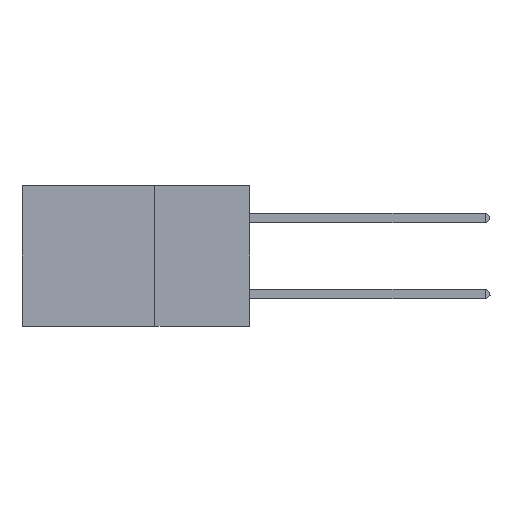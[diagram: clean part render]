
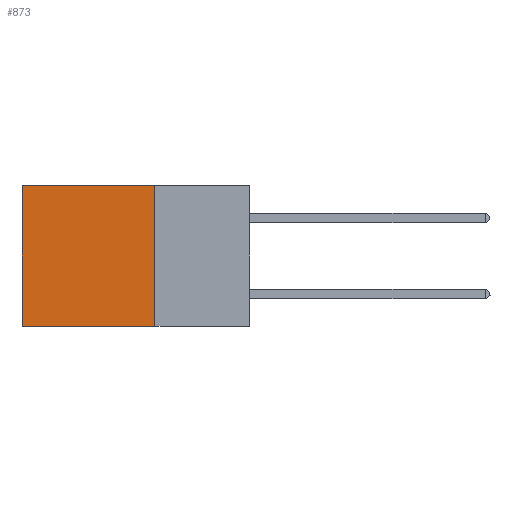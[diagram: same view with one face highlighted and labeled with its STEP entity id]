
A CAD part, left-side view. The second image highlights one B-rep face of the part: STEP entity #873.
In plain terms, the highlighted planar face has unit normal (-1, 0, 0).
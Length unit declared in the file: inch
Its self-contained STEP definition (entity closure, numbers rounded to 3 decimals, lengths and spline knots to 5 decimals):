
#191 = EDGE_LOOP ( 'NONE', ( #27006, #25550, #25940, #15339 ) ) ;
#236 = VECTOR ( 'NONE', #26008, 39.37008 ) ;
#326 = VERTEX_POINT ( 'NONE', #21121 ) ;
#873 = ADVANCED_FACE ( 'NONE', ( #15754 ), #25463, .F. ) ;
#1130 = VECTOR ( 'NONE', #25966, 39.37008 ) ;
#1769 = VECTOR ( 'NONE', #19743, 39.37008 ) ;
#2538 = CARTESIAN_POINT ( 'NONE',  ( 0.2875, 0.25, -0.37 ) ) ;
#9728 = VECTOR ( 'NONE', #25438, 39.37008 ) ;
#10364 = CARTESIAN_POINT ( 'NONE',  ( 0.2875, 0.25, 0. ) ) ;
#10390 = CARTESIAN_POINT ( 'NONE',  ( 0.2875, 0.25, 0. ) ) ;
#10706 = DIRECTION ( 'NONE',  ( 1., 0., 0. ) ) ;
#10878 = LINE ( 'NONE', #10364, #9728 ) ;
#11114 = CARTESIAN_POINT ( 'NONE',  ( 0.2875, 0.25, 0. ) ) ;
#12013 = CARTESIAN_POINT ( 'NONE',  ( 0.2875, 0.6, 0. ) ) ;
#12786 = EDGE_CURVE ( 'NONE', #13239, #17150, #27253, .T. ) ;
#13200 = EDGE_CURVE ( 'NONE', #13239, #31887, #10878, .T. ) ;
#13239 = VERTEX_POINT ( 'NONE', #27892 ) ;
#13364 = CARTESIAN_POINT ( 'NONE',  ( 0.2875, 0.25, -0.37 ) ) ;
#14300 = EDGE_CURVE ( 'NONE', #31887, #326, #20175, .T. ) ;
#15339 = ORIENTED_EDGE ( 'NONE', *, *, #12786, .T. ) ;
#15754 = FACE_OUTER_BOUND ( 'NONE', #191, .T. ) ;
#17150 = VERTEX_POINT ( 'NONE', #21520 ) ;
#19743 = DIRECTION ( 'NONE',  ( 0., 0., -1. ) ) ;
#20175 = LINE ( 'NONE', #13364, #236 ) ;
#21121 = CARTESIAN_POINT ( 'NONE',  ( 0.2875, 0.6, -0.37 ) ) ;
#21520 = CARTESIAN_POINT ( 'NONE',  ( 0.2875, 0.6, 0. ) ) ;
#22091 = EDGE_CURVE ( 'NONE', #17150, #326, #31461, .T. ) ;
#25438 = DIRECTION ( 'NONE',  ( 0., 0., -1. ) ) ;
#25463 = PLANE ( 'NONE',  #31323 ) ;
#25550 = ORIENTED_EDGE ( 'NONE', *, *, #14300, .F. ) ;
#25940 = ORIENTED_EDGE ( 'NONE', *, *, #13200, .F. ) ;
#25966 = DIRECTION ( 'NONE',  ( 0., 1., 0. ) ) ;
#26008 = DIRECTION ( 'NONE',  ( 0., 1., 0. ) ) ;
#27006 = ORIENTED_EDGE ( 'NONE', *, *, #22091, .T. ) ;
#27253 = LINE ( 'NONE', #11114, #1130 ) ;
#27892 = CARTESIAN_POINT ( 'NONE',  ( 0.2875, 0.25, 0. ) ) ;
#30678 = DIRECTION ( 'NONE',  ( 0., 0., -1. ) ) ;
#31323 = AXIS2_PLACEMENT_3D ( 'NONE', #10390, #10706, #30678 ) ;
#31461 = LINE ( 'NONE', #12013, #1769 ) ;
#31887 = VERTEX_POINT ( 'NONE', #2538 ) ;
